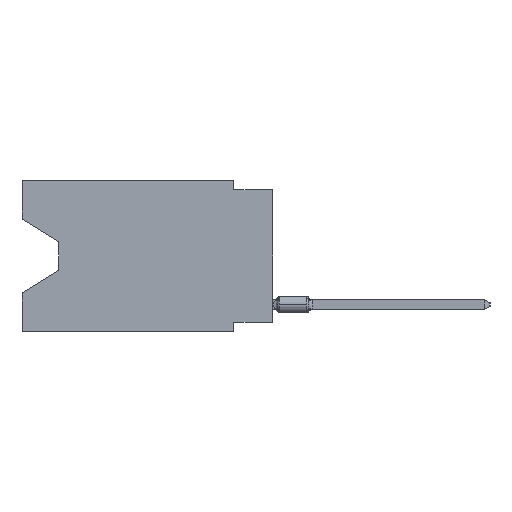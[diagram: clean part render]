
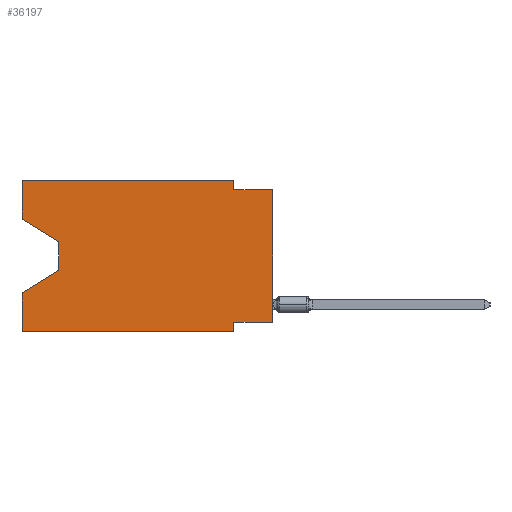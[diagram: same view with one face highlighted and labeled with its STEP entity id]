
A CAD part, left-side view. The second image highlights one B-rep face of the part: STEP entity #36197.
In plain terms, the highlighted planar face has unit normal (-1, 0, 0).
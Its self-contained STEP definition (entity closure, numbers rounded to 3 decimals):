
#679 = DIRECTION ( 'NONE',  ( 0., 1., 0. ) ) ;
#2617 = ORIENTED_EDGE ( 'NONE', *, *, #28355, .F. ) ;
#2986 = ORIENTED_EDGE ( 'NONE', *, *, #34164, .F. ) ;
#3030 = VERTEX_POINT ( 'NONE', #47971 ) ;
#3555 = EDGE_CURVE ( 'NONE', #42598, #13571, #26007, .T. ) ;
#4843 = VECTOR ( 'NONE', #22920, 1000. ) ;
#5838 = CARTESIAN_POINT ( 'NONE',  ( 0., 13.97, -4.013 ) ) ;
#6550 = ORIENTED_EDGE ( 'NONE', *, *, #20543, .F. ) ;
#7404 = CARTESIAN_POINT ( 'NONE',  ( 0., 2.54, 0. ) ) ;
#7519 = DIRECTION ( 'NONE',  ( 0., 0., 1. ) ) ;
#7861 = VERTEX_POINT ( 'NONE', #15133 ) ;
#8225 = LINE ( 'NONE', #31394, #23045 ) ;
#8257 = ORIENTED_EDGE ( 'NONE', *, *, #3555, .T. ) ;
#8458 = LINE ( 'NONE', #20828, #22912 ) ;
#9110 = LINE ( 'NONE', #5838, #41720 ) ;
#11148 = EDGE_CURVE ( 'NONE', #49741, #43831, #31603, .T. ) ;
#11926 = LINE ( 'NONE', #7404, #23077 ) ;
#12990 = DIRECTION ( 'NONE',  ( 0., -1., 0. ) ) ;
#13046 = DIRECTION ( 'NONE',  ( 0., 0.855, -0.519 ) ) ;
#13571 = VERTEX_POINT ( 'NONE', #42067 ) ;
#14214 = CARTESIAN_POINT ( 'NONE',  ( 0., 16.383, 0. ) ) ;
#14605 = CARTESIAN_POINT ( 'NONE',  ( 0., 13.97, -5.893 ) ) ;
#14653 = EDGE_CURVE ( 'NONE', #42598, #15807, #8225, .T. ) ;
#15133 = CARTESIAN_POINT ( 'NONE',  ( 0., 13.97, -4.013 ) ) ;
#15154 = VECTOR ( 'NONE', #23665, 1000. ) ;
#15807 = VERTEX_POINT ( 'NONE', #22959 ) ;
#16349 = CARTESIAN_POINT ( 'NONE',  ( 0., 16.383, -9.906 ) ) ;
#16424 = DIRECTION ( 'NONE',  ( 0., 0., -1. ) ) ;
#16457 = CARTESIAN_POINT ( 'NONE',  ( 0., 16.383, -9.906 ) ) ;
#18059 = LINE ( 'NONE', #38179, #33548 ) ;
#18263 = DIRECTION ( 'NONE',  ( 0., 0., -1. ) ) ;
#18377 = LINE ( 'NONE', #18884, #4843 ) ;
#18884 = CARTESIAN_POINT ( 'NONE',  ( 0., 0., -0.635 ) ) ;
#19515 = DIRECTION ( 'NONE',  ( 0., 0., -1. ) ) ;
#19992 = VECTOR ( 'NONE', #7519, 1000. ) ;
#20359 = VECTOR ( 'NONE', #31359, 1000. ) ;
#20543 = EDGE_CURVE ( 'NONE', #40208, #49517, #11926, .T. ) ;
#20828 = CARTESIAN_POINT ( 'NONE',  ( 0., 16.383, 0. ) ) ;
#21379 = EDGE_LOOP ( 'NONE', ( #40321, #43491, #26443, #2986, #32141, #37076, #48362, #8257, #38334, #6550, #2617, #38978 ) ) ;
#21873 = EDGE_CURVE ( 'NONE', #15807, #37174, #18059, .T. ) ;
#22145 = CARTESIAN_POINT ( 'NONE',  ( 0., 2.54, -0.635 ) ) ;
#22520 = EDGE_CURVE ( 'NONE', #7861, #3030, #9110, .T. ) ;
#22912 = VECTOR ( 'NONE', #12990, 1000. ) ;
#22920 = DIRECTION ( 'NONE',  ( 0., -1., 0. ) ) ;
#22959 = CARTESIAN_POINT ( 'NONE',  ( 0., 2.54, -9.271 ) ) ;
#23045 = VECTOR ( 'NONE', #679, 1000. ) ;
#23077 = VECTOR ( 'NONE', #19515, 1000. ) ;
#23407 = LINE ( 'NONE', #42048, #33314 ) ;
#23665 = DIRECTION ( 'NONE',  ( 0., 0., 1. ) ) ;
#23769 = EDGE_CURVE ( 'NONE', #49517, #13571, #18377, .T. ) ;
#23819 = CARTESIAN_POINT ( 'NONE',  ( 0., 16.383, 0. ) ) ;
#25648 = VERTEX_POINT ( 'NONE', #49569 ) ;
#26007 = LINE ( 'NONE', #31448, #15154 ) ;
#26443 = ORIENTED_EDGE ( 'NONE', *, *, #38539, .T. ) ;
#26559 = CARTESIAN_POINT ( 'NONE',  ( 0., 0., -9.271 ) ) ;
#28355 = EDGE_CURVE ( 'NONE', #43831, #40208, #8458, .T. ) ;
#31359 = DIRECTION ( 'NONE',  ( 0., 0., 1. ) ) ;
#31373 = AXIS2_PLACEMENT_3D ( 'NONE', #14214, #48210, #18263 ) ;
#31394 = CARTESIAN_POINT ( 'NONE',  ( 0., 0., -9.271 ) ) ;
#31448 = CARTESIAN_POINT ( 'NONE',  ( 0., 0., 0. ) ) ;
#31467 = LINE ( 'NONE', #16349, #34675 ) ;
#31603 = LINE ( 'NONE', #23819, #20359 ) ;
#32141 = ORIENTED_EDGE ( 'NONE', *, *, #48027, .T. ) ;
#32651 = CARTESIAN_POINT ( 'NONE',  ( 0., 16.383, -2.546 ) ) ;
#33228 = LINE ( 'NONE', #45059, #19992 ) ;
#33314 = VECTOR ( 'NONE', #38012, 1000. ) ;
#33548 = VECTOR ( 'NONE', #37679, 1000. ) ;
#34164 = EDGE_CURVE ( 'NONE', #47111, #25648, #33228, .T. ) ;
#34675 = VECTOR ( 'NONE', #47062, 1000. ) ;
#36197 = ADVANCED_FACE ( 'NONE', ( #43952 ), #48707, .F. ) ;
#36494 = VECTOR ( 'NONE', #13046, 1000. ) ;
#37076 = ORIENTED_EDGE ( 'NONE', *, *, #21873, .F. ) ;
#37174 = VERTEX_POINT ( 'NONE', #45524 ) ;
#37679 = DIRECTION ( 'NONE',  ( 0., 0., -1. ) ) ;
#38012 = DIRECTION ( 'NONE',  ( 0., -0.855, -0.519 ) ) ;
#38179 = CARTESIAN_POINT ( 'NONE',  ( 0., 2.54, -9.906 ) ) ;
#38334 = ORIENTED_EDGE ( 'NONE', *, *, #23769, .F. ) ;
#38539 = EDGE_CURVE ( 'NONE', #3030, #25648, #49104, .T. ) ;
#38676 = CARTESIAN_POINT ( 'NONE',  ( 0., 16.383, 0. ) ) ;
#38978 = ORIENTED_EDGE ( 'NONE', *, *, #11148, .F. ) ;
#40208 = VERTEX_POINT ( 'NONE', #42347 ) ;
#40321 = ORIENTED_EDGE ( 'NONE', *, *, #40623, .T. ) ;
#40623 = EDGE_CURVE ( 'NONE', #49741, #7861, #23407, .T. ) ;
#41720 = VECTOR ( 'NONE', #16424, 1000. ) ;
#42048 = CARTESIAN_POINT ( 'NONE',  ( 0., 16.383, -2.546 ) ) ;
#42067 = CARTESIAN_POINT ( 'NONE',  ( 0., 0., -0.635 ) ) ;
#42347 = CARTESIAN_POINT ( 'NONE',  ( 0., 2.54, 0. ) ) ;
#42598 = VERTEX_POINT ( 'NONE', #26559 ) ;
#43491 = ORIENTED_EDGE ( 'NONE', *, *, #22520, .T. ) ;
#43831 = VERTEX_POINT ( 'NONE', #38676 ) ;
#43952 = FACE_OUTER_BOUND ( 'NONE', #21379, .T. ) ;
#45059 = CARTESIAN_POINT ( 'NONE',  ( 0., 16.383, 0. ) ) ;
#45524 = CARTESIAN_POINT ( 'NONE',  ( 0., 2.54, -9.906 ) ) ;
#47062 = DIRECTION ( 'NONE',  ( 0., -1., 0. ) ) ;
#47111 = VERTEX_POINT ( 'NONE', #16457 ) ;
#47971 = CARTESIAN_POINT ( 'NONE',  ( 0., 13.97, -5.893 ) ) ;
#48027 = EDGE_CURVE ( 'NONE', #47111, #37174, #31467, .T. ) ;
#48210 = DIRECTION ( 'NONE',  ( 1., 0., 0. ) ) ;
#48362 = ORIENTED_EDGE ( 'NONE', *, *, #14653, .F. ) ;
#48707 = PLANE ( 'NONE',  #31373 ) ;
#49104 = LINE ( 'NONE', #14605, #36494 ) ;
#49517 = VERTEX_POINT ( 'NONE', #22145 ) ;
#49569 = CARTESIAN_POINT ( 'NONE',  ( 0., 16.383, -7.36 ) ) ;
#49741 = VERTEX_POINT ( 'NONE', #32651 ) ;
